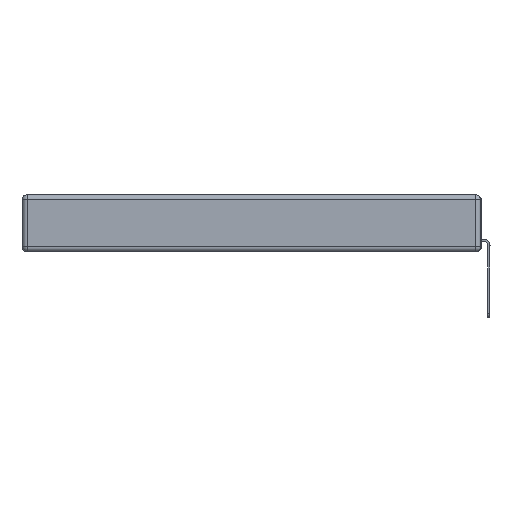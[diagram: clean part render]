
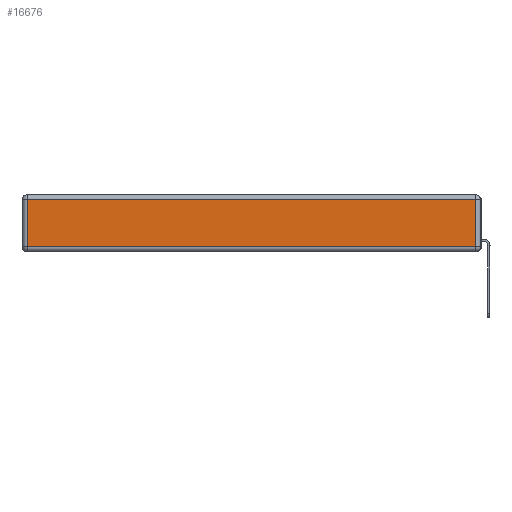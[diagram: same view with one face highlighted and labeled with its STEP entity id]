
A CAD part, left-side view. The second image highlights one B-rep face of the part: STEP entity #16676.
In plain terms, the highlighted planar face has unit normal (-1, 0, 0).
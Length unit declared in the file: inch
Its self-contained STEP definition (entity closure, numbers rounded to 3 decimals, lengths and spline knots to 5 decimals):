
#1300 = DIRECTION ( 'NONE',  ( -1., 0., 0. ) ) ;
#1473 = CARTESIAN_POINT ( 'NONE',  ( 0., 0.03, -0.03 ) ) ;
#1907 = DIRECTION ( 'NONE',  ( 0., -1., 0. ) ) ;
#1960 = VERTEX_POINT ( 'NONE', #1473 ) ;
#2220 = DIRECTION ( 'NONE',  ( 0., 0., -1. ) ) ;
#2933 = VERTEX_POINT ( 'NONE', #17789 ) ;
#3074 = VECTOR ( 'NONE', #12249, 39.37008 ) ;
#3134 = EDGE_CURVE ( 'NONE', #11083, #11901, #19769, .T. ) ;
#3149 = LINE ( 'NONE', #19046, #10671 ) ;
#4216 = DIRECTION ( 'NONE',  ( 0., 0., 1. ) ) ;
#4317 = CARTESIAN_POINT ( 'NONE',  ( 0., 0., -0.343 ) ) ;
#4374 = CARTESIAN_POINT ( 'NONE',  ( 0., 0.03, -0.343 ) ) ;
#5555 = CARTESIAN_POINT ( 'NONE',  ( 0., 2.72, -0.03 ) ) ;
#5632 = LINE ( 'NONE', #4374, #3074 ) ;
#7342 = CARTESIAN_POINT ( 'NONE',  ( 0., 2.72, -0.313 ) ) ;
#9007 = AXIS2_PLACEMENT_3D ( 'NONE', #4317, #1300, #4216 ) ;
#9923 = DIRECTION ( 'NONE',  ( 0., 1., 0. ) ) ;
#10671 = VECTOR ( 'NONE', #1907, 39.37008 ) ;
#10700 = VECTOR ( 'NONE', #9923, 39.37008 ) ;
#11083 = VERTEX_POINT ( 'NONE', #5555 ) ;
#11661 = ORIENTED_EDGE ( 'NONE', *, *, #16471, .T. ) ;
#11745 = CARTESIAN_POINT ( 'NONE',  ( 0., 2.72, -0.343 ) ) ;
#11846 = ORIENTED_EDGE ( 'NONE', *, *, #17338, .T. ) ;
#11901 = VERTEX_POINT ( 'NONE', #7342 ) ;
#12249 = DIRECTION ( 'NONE',  ( 0., 0., 1. ) ) ;
#13699 = EDGE_LOOP ( 'NONE', ( #11846, #19033, #11661, #18070 ) ) ;
#14500 = CARTESIAN_POINT ( 'NONE',  ( 0., 2.75, -0.03 ) ) ;
#15529 = FACE_OUTER_BOUND ( 'NONE', #13699, .T. ) ;
#16055 = LINE ( 'NONE', #14500, #10700 ) ;
#16471 = EDGE_CURVE ( 'NONE', #1960, #11083, #16055, .T. ) ;
#16605 = VECTOR ( 'NONE', #2220, 39.37008 ) ;
#16676 = ADVANCED_FACE ( 'NONE', ( #15529 ), #20323, .T. ) ;
#17338 = EDGE_CURVE ( 'NONE', #11901, #2933, #3149, .T. ) ;
#17637 = EDGE_CURVE ( 'NONE', #2933, #1960, #5632, .T. ) ;
#17789 = CARTESIAN_POINT ( 'NONE',  ( 0., 0.03, -0.313 ) ) ;
#18070 = ORIENTED_EDGE ( 'NONE', *, *, #3134, .T. ) ;
#19033 = ORIENTED_EDGE ( 'NONE', *, *, #17637, .T. ) ;
#19046 = CARTESIAN_POINT ( 'NONE',  ( 0., 0., -0.313 ) ) ;
#19769 = LINE ( 'NONE', #11745, #16605 ) ;
#20323 = PLANE ( 'NONE',  #9007 ) ;
